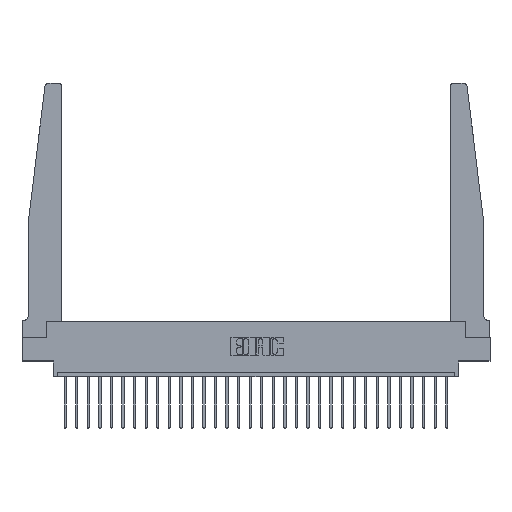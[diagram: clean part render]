
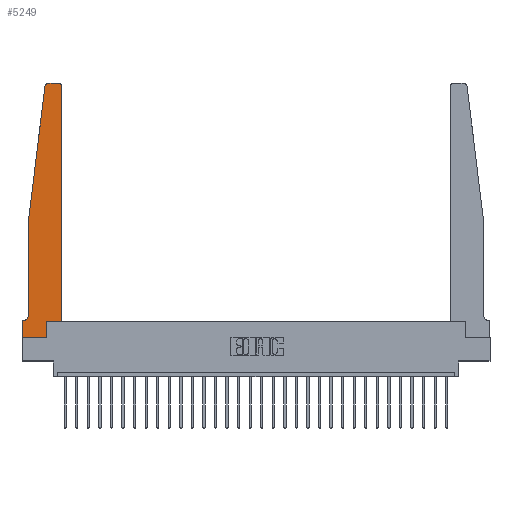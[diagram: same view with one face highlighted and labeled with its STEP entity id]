
A CAD part, top view. The second image highlights one B-rep face of the part: STEP entity #5249.
In plain terms, the highlighted planar face has unit normal (0, 0, 1).
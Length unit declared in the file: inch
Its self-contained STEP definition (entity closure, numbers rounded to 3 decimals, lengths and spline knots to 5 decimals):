
#423 = LINE ( 'NONE', #23367, #13232 ) ;
#556 = VERTEX_POINT ( 'NONE', #20227 ) ;
#724 = DIRECTION ( 'NONE',  ( 1., 0., 0. ) ) ;
#970 = LINE ( 'NONE', #25252, #22250 ) ;
#1171 = CARTESIAN_POINT ( 'NONE',  ( 0., 0., 0.37 ) ) ;
#1260 = AXIS2_PLACEMENT_3D ( 'NONE', #21059, #25333, #2415 ) ;
#1371 = CARTESIAN_POINT ( 'NONE',  ( 0.2605, 0.18, 0.37 ) ) ;
#2415 = DIRECTION ( 'NONE',  ( -1., 0., 0. ) ) ;
#2609 = DIRECTION ( 'NONE',  ( -1., 0., 0. ) ) ;
#2717 = CARTESIAN_POINT ( 'NONE',  ( 0.395, 2.72, 0.37 ) ) ;
#3077 = CARTESIAN_POINT ( 'NONE',  ( 0.2605, 0.18, 0.37 ) ) ;
#3351 = DIRECTION ( 'NONE',  ( 1., 0., 0. ) ) ;
#3391 = EDGE_LOOP ( 'NONE', ( #5700, #10553, #18477, #24642, #7392, #18527, #18121, #11605, #24715, #26668, #4929, #23714 ) ) ;
#4162 = EDGE_CURVE ( 'NONE', #22750, #11643, #18739, .T. ) ;
#4439 = VERTEX_POINT ( 'NONE', #23034 ) ;
#4481 = CARTESIAN_POINT ( 'NONE',  ( 0., 0.1875, 0.37 ) ) ;
#4812 = VERTEX_POINT ( 'NONE', #19736 ) ;
#4899 = LINE ( 'NONE', #7416, #15429 ) ;
#4929 = ORIENTED_EDGE ( 'NONE', *, *, #14020, .T. ) ;
#5054 = DIRECTION ( 'NONE',  ( 1., 0., 0. ) ) ;
#5122 = LINE ( 'NONE', #23742, #16583 ) ;
#5249 = ADVANCED_FACE ( 'NONE', ( #19333 ), #19381, .T. ) ;
#5269 = CIRCLE ( 'NONE', #1260, 0.05 ) ;
#5432 = DIRECTION ( 'NONE',  ( 0., -1., 0. ) ) ;
#5503 = AXIS2_PLACEMENT_3D ( 'NONE', #4481, #10933, #21410 ) ;
#5700 = ORIENTED_EDGE ( 'NONE', *, *, #14331, .T. ) ;
#5713 = CARTESIAN_POINT ( 'NONE',  ( 0., 0., 0.37 ) ) ;
#6094 = DIRECTION ( 'NONE',  ( 0., 1., 0. ) ) ;
#6495 = EDGE_CURVE ( 'NONE', #18323, #4439, #970, .T. ) ;
#6725 = AXIS2_PLACEMENT_3D ( 'NONE', #2717, #25572, #724 ) ;
#7025 = CIRCLE ( 'NONE', #6725, 0.03 ) ;
#7392 = ORIENTED_EDGE ( 'NONE', *, *, #14809, .T. ) ;
#7416 = CARTESIAN_POINT ( 'NONE',  ( 0.065, 1.25, 0.37 ) ) ;
#7609 = VERTEX_POINT ( 'NONE', #19826 ) ;
#7626 = CARTESIAN_POINT ( 'NONE',  ( 0.425, 0.18, 0.37 ) ) ;
#8040 = CARTESIAN_POINT ( 'NONE',  ( 0.425, 0.18, 0.37 ) ) ;
#8281 = VECTOR ( 'NONE', #17631, 39.37008 ) ;
#9138 = EDGE_CURVE ( 'NONE', #17080, #556, #4899, .T. ) ;
#9528 = AXIS2_PLACEMENT_3D ( 'NONE', #17866, #9566, #5054 ) ;
#9566 = DIRECTION ( 'NONE',  ( 0., 0., 1. ) ) ;
#10208 = CARTESIAN_POINT ( 'NONE',  ( 0.425, 2.72, 0.37 ) ) ;
#10362 = VERTEX_POINT ( 'NONE', #14136 ) ;
#10553 = ORIENTED_EDGE ( 'NONE', *, *, #4162, .T. ) ;
#10708 = VERTEX_POINT ( 'NONE', #7626 ) ;
#10933 = DIRECTION ( 'NONE',  ( 0., 0., 1. ) ) ;
#10976 = EDGE_CURVE ( 'NONE', #19123, #10708, #5122, .T. ) ;
#11244 = LINE ( 'NONE', #5713, #16458 ) ;
#11605 = ORIENTED_EDGE ( 'NONE', *, *, #24852, .T. ) ;
#11643 = VERTEX_POINT ( 'NONE', #19309 ) ;
#12040 = VECTOR ( 'NONE', #20488, 39.37008 ) ;
#13232 = VECTOR ( 'NONE', #2609, 39.37008 ) ;
#13727 = VERTEX_POINT ( 'NONE', #10208 ) ;
#14020 = EDGE_CURVE ( 'NONE', #10708, #13727, #25266, .T. ) ;
#14136 = CARTESIAN_POINT ( 'NONE',  ( 0.395, 2.75, 0.37 ) ) ;
#14331 = EDGE_CURVE ( 'NONE', #10362, #22750, #423, .T. ) ;
#14564 = LINE ( 'NONE', #1171, #18099 ) ;
#14809 = EDGE_CURVE ( 'NONE', #556, #18323, #5269, .T. ) ;
#15429 = VECTOR ( 'NONE', #16490, 39.37008 ) ;
#15860 = LINE ( 'NONE', #3077, #8281 ) ;
#16458 = VECTOR ( 'NONE', #5432, 39.37008 ) ;
#16490 = DIRECTION ( 'NONE',  ( 0., -1., 0. ) ) ;
#16583 = VECTOR ( 'NONE', #3351, 39.37008 ) ;
#17080 = VERTEX_POINT ( 'NONE', #19474 ) ;
#17587 = CARTESIAN_POINT ( 'NONE',  ( 0.27653, 2.75, 0.37 ) ) ;
#17631 = DIRECTION ( 'NONE',  ( 0., 1., 0. ) ) ;
#17739 = EDGE_CURVE ( 'NONE', #13727, #10362, #7025, .T. ) ;
#17866 = CARTESIAN_POINT ( 'NONE',  ( 0.27653, 2.72, 0.37 ) ) ;
#18099 = VECTOR ( 'NONE', #22209, 39.37008 ) ;
#18121 = ORIENTED_EDGE ( 'NONE', *, *, #25336, .T. ) ;
#18311 = CARTESIAN_POINT ( 'NONE',  ( 0.065, 1.25, 0.37 ) ) ;
#18323 = VERTEX_POINT ( 'NONE', #24524 ) ;
#18477 = ORIENTED_EDGE ( 'NONE', *, *, #22991, .T. ) ;
#18527 = ORIENTED_EDGE ( 'NONE', *, *, #6495, .T. ) ;
#18739 = CIRCLE ( 'NONE', #9528, 0.03 ) ;
#19123 = VERTEX_POINT ( 'NONE', #1371 ) ;
#19309 = CARTESIAN_POINT ( 'NONE',  ( 0.24675, 2.72367, 0.37 ) ) ;
#19333 = FACE_OUTER_BOUND ( 'NONE', #3391, .T. ) ;
#19381 = PLANE ( 'NONE',  #5503 ) ;
#19474 = CARTESIAN_POINT ( 'NONE',  ( 0.065, 1.25, 0.37 ) ) ;
#19713 = VECTOR ( 'NONE', #6094, 39.37008 ) ;
#19736 = CARTESIAN_POINT ( 'NONE',  ( 0.2605, 0., 0.37 ) ) ;
#19826 = CARTESIAN_POINT ( 'NONE',  ( 0., 0., 0.37 ) ) ;
#20227 = CARTESIAN_POINT ( 'NONE',  ( 0.065, 0.2375, 0.37 ) ) ;
#20488 = DIRECTION ( 'NONE',  ( -0.122, -0.992, 0. ) ) ;
#21059 = CARTESIAN_POINT ( 'NONE',  ( 0.015, 0.2375, 0.37 ) ) ;
#21135 = LINE ( 'NONE', #18311, #12040 ) ;
#21410 = DIRECTION ( 'NONE',  ( 1., 0., 0. ) ) ;
#22209 = DIRECTION ( 'NONE',  ( 1., 0., 0. ) ) ;
#22250 = VECTOR ( 'NONE', #25432, 39.37008 ) ;
#22750 = VERTEX_POINT ( 'NONE', #17587 ) ;
#22991 = EDGE_CURVE ( 'NONE', #11643, #17080, #21135, .T. ) ;
#23034 = CARTESIAN_POINT ( 'NONE',  ( 0., 0.1875, 0.37 ) ) ;
#23367 = CARTESIAN_POINT ( 'NONE',  ( 0.25, 2.75, 0.37 ) ) ;
#23714 = ORIENTED_EDGE ( 'NONE', *, *, #17739, .T. ) ;
#23742 = CARTESIAN_POINT ( 'NONE',  ( 0.425, 0.18, 0.37 ) ) ;
#24524 = CARTESIAN_POINT ( 'NONE',  ( 0.015, 0.1875, 0.37 ) ) ;
#24642 = ORIENTED_EDGE ( 'NONE', *, *, #9138, .T. ) ;
#24715 = ORIENTED_EDGE ( 'NONE', *, *, #24776, .T. ) ;
#24776 = EDGE_CURVE ( 'NONE', #4812, #19123, #15860, .T. ) ;
#24852 = EDGE_CURVE ( 'NONE', #7609, #4812, #14564, .T. ) ;
#25252 = CARTESIAN_POINT ( 'NONE',  ( 0.065, 0.1875, 0.37 ) ) ;
#25266 = LINE ( 'NONE', #8040, #19713 ) ;
#25333 = DIRECTION ( 'NONE',  ( 0., 0., -1. ) ) ;
#25336 = EDGE_CURVE ( 'NONE', #4439, #7609, #11244, .T. ) ;
#25432 = DIRECTION ( 'NONE',  ( -1., 0., 0. ) ) ;
#25572 = DIRECTION ( 'NONE',  ( 0., 0., 1. ) ) ;
#26668 = ORIENTED_EDGE ( 'NONE', *, *, #10976, .T. ) ;
